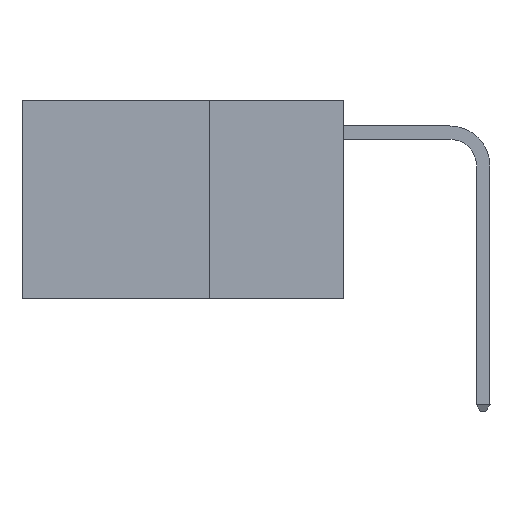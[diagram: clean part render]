
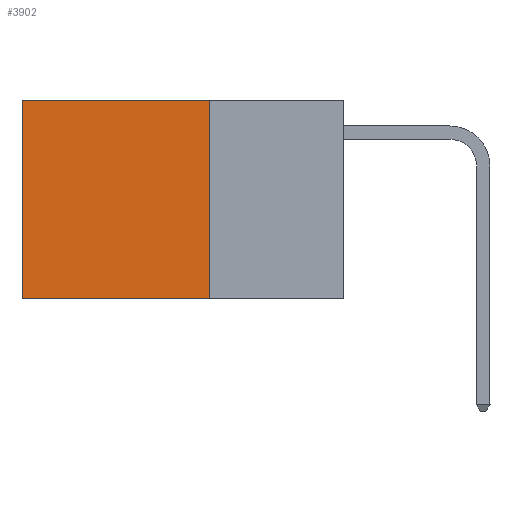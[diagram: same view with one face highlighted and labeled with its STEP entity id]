
A CAD part, left-side view. The second image highlights one B-rep face of the part: STEP entity #3902.
In plain terms, the highlighted planar face has unit normal (-1, 0, 0).
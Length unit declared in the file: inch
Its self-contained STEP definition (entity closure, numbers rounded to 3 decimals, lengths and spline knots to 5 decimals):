
#33 = LINE ( 'NONE', #10509, #2252 ) ;
#207 = FACE_OUTER_BOUND ( 'NONE', #9930, .T. ) ;
#1650 = EDGE_CURVE ( 'NONE', #9575, #15698, #15366, .T. ) ;
#2186 = VECTOR ( 'NONE', #17600, 39.37008 ) ;
#2252 = VECTOR ( 'NONE', #21131, 39.37008 ) ;
#2424 = EDGE_CURVE ( 'NONE', #19411, #2926, #20063, .T. ) ;
#2926 = VERTEX_POINT ( 'NONE', #7584 ) ;
#3902 = ADVANCED_FACE ( 'NONE', ( #207 ), #23703, .F. ) ;
#6354 = DIRECTION ( 'NONE',  ( 1., 0., 0. ) ) ;
#6425 = CARTESIAN_POINT ( 'NONE',  ( 0.2625, 0.25, 0. ) ) ;
#7204 = DIRECTION ( 'NONE',  ( 0., 0., -1. ) ) ;
#7379 = VECTOR ( 'NONE', #7204, 39.37008 ) ;
#7584 = CARTESIAN_POINT ( 'NONE',  ( 0.2625, 0.6, -0.37 ) ) ;
#9271 = CARTESIAN_POINT ( 'NONE',  ( 0.2625, 0.25, -0.37 ) ) ;
#9575 = VERTEX_POINT ( 'NONE', #21834 ) ;
#9930 = EDGE_LOOP ( 'NONE', ( #25071, #19737, #21700, #18848 ) ) ;
#10070 = CARTESIAN_POINT ( 'NONE',  ( 0.2625, 0.6, 0. ) ) ;
#10509 = CARTESIAN_POINT ( 'NONE',  ( 0.2625, 0.25, -0.37 ) ) ;
#13030 = EDGE_CURVE ( 'NONE', #15698, #2926, #33, .T. ) ;
#13454 = EDGE_CURVE ( 'NONE', #9575, #19411, #18884, .T. ) ;
#14301 = AXIS2_PLACEMENT_3D ( 'NONE', #25650, #6354, #17119 ) ;
#15366 = LINE ( 'NONE', #6425, #2186 ) ;
#15698 = VERTEX_POINT ( 'NONE', #9271 ) ;
#17119 = DIRECTION ( 'NONE',  ( 0., 0., -1. ) ) ;
#17600 = DIRECTION ( 'NONE',  ( 0., 0., -1. ) ) ;
#17913 = VECTOR ( 'NONE', #20969, 39.37008 ) ;
#18848 = ORIENTED_EDGE ( 'NONE', *, *, #13454, .T. ) ;
#18884 = LINE ( 'NONE', #23078, #17913 ) ;
#19411 = VERTEX_POINT ( 'NONE', #10070 ) ;
#19737 = ORIENTED_EDGE ( 'NONE', *, *, #13030, .F. ) ;
#20063 = LINE ( 'NONE', #22026, #7379 ) ;
#20969 = DIRECTION ( 'NONE',  ( 0., 1., 0. ) ) ;
#21131 = DIRECTION ( 'NONE',  ( 0., 1., 0. ) ) ;
#21700 = ORIENTED_EDGE ( 'NONE', *, *, #1650, .F. ) ;
#21834 = CARTESIAN_POINT ( 'NONE',  ( 0.2625, 0.25, 0. ) ) ;
#22026 = CARTESIAN_POINT ( 'NONE',  ( 0.2625, 0.6, 0. ) ) ;
#23078 = CARTESIAN_POINT ( 'NONE',  ( 0.2625, 0.25, 0. ) ) ;
#23703 = PLANE ( 'NONE',  #14301 ) ;
#25071 = ORIENTED_EDGE ( 'NONE', *, *, #2424, .T. ) ;
#25650 = CARTESIAN_POINT ( 'NONE',  ( 0.2625, 0.25, 0. ) ) ;
